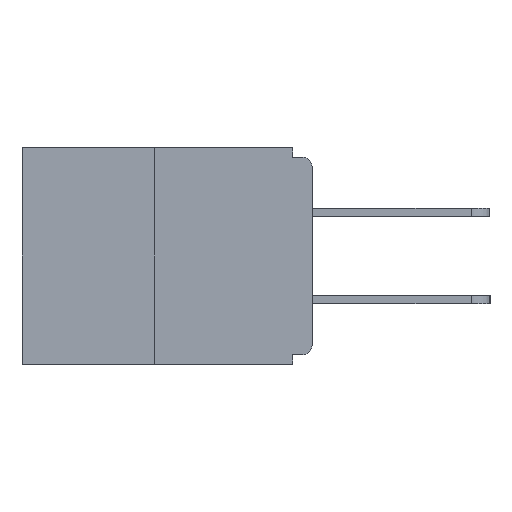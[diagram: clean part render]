
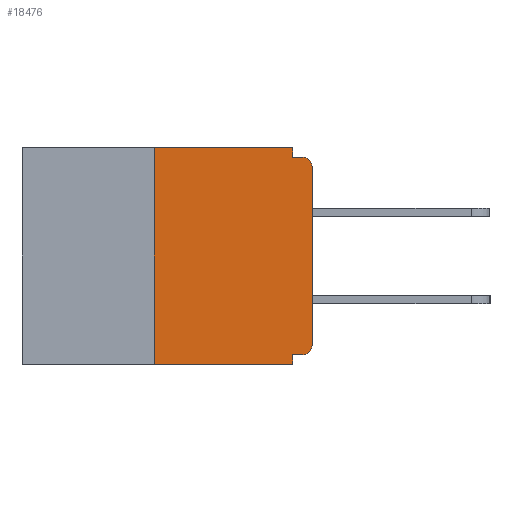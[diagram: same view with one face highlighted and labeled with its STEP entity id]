
A CAD part, left-side view. The second image highlights one B-rep face of the part: STEP entity #18476.
In plain terms, the highlighted planar face has unit normal (-1, 0, 0).
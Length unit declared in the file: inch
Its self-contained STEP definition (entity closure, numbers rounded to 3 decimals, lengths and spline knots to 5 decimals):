
#131 = EDGE_CURVE ( 'NONE', #29105, #17084, #5404, .T. ) ;
#136 = CARTESIAN_POINT ( 'NONE',  ( 0., 0.031, -0.343 ) ) ;
#494 = EDGE_CURVE ( 'NONE', #11780, #4640, #24787, .T. ) ;
#502 = VERTEX_POINT ( 'NONE', #136 ) ;
#1142 = CARTESIAN_POINT ( 'NONE',  ( 0., 0.25, -0.343 ) ) ;
#2443 = VECTOR ( 'NONE', #16193, 39.37008 ) ;
#2711 = CIRCLE ( 'NONE', #31239, 0.015 ) ;
#2719 = AXIS2_PLACEMENT_3D ( 'NONE', #22281, #15550, #10317 ) ;
#2957 = CARTESIAN_POINT ( 'NONE',  ( 0., 0.015, -0.015 ) ) ;
#4151 = VERTEX_POINT ( 'NONE', #19527 ) ;
#4197 = DIRECTION ( 'NONE',  ( 0., 1., 0. ) ) ;
#4585 = LINE ( 'NONE', #31349, #31183 ) ;
#4640 = VERTEX_POINT ( 'NONE', #27849 ) ;
#5404 = LINE ( 'NONE', #24868, #15585 ) ;
#5743 = ORIENTED_EDGE ( 'NONE', *, *, #494, .T. ) ;
#6564 = EDGE_CURVE ( 'NONE', #17084, #4151, #4585, .T. ) ;
#6596 = EDGE_CURVE ( 'NONE', #4640, #14128, #23706, .T. ) ;
#6706 = VERTEX_POINT ( 'NONE', #2957 ) ;
#7987 = VECTOR ( 'NONE', #19180, 39.37008 ) ;
#8022 = ORIENTED_EDGE ( 'NONE', *, *, #24861, .F. ) ;
#8413 = CARTESIAN_POINT ( 'NONE',  ( 0., 0., -0.03 ) ) ;
#8784 = ORIENTED_EDGE ( 'NONE', *, *, #8794, .T. ) ;
#8794 = EDGE_CURVE ( 'NONE', #19046, #502, #14116, .T. ) ;
#9097 = ORIENTED_EDGE ( 'NONE', *, *, #11865, .T. ) ;
#9131 = CARTESIAN_POINT ( 'NONE',  ( 0., 0.031, -0.343 ) ) ;
#10240 = DIRECTION ( 'NONE',  ( 0., 0., -1. ) ) ;
#10317 = DIRECTION ( 'NONE',  ( 0., 0., -1. ) ) ;
#11246 = VERTEX_POINT ( 'NONE', #11275 ) ;
#11275 = CARTESIAN_POINT ( 'NONE',  ( 0., 0.031, -0.328 ) ) ;
#11780 = VERTEX_POINT ( 'NONE', #12622 ) ;
#11865 = EDGE_CURVE ( 'NONE', #14128, #6706, #2711, .T. ) ;
#12084 = DIRECTION ( 'NONE',  ( -1., 0., 0. ) ) ;
#12622 = CARTESIAN_POINT ( 'NONE',  ( 0., 0.015, -0.328 ) ) ;
#13083 = VECTOR ( 'NONE', #30305, 39.37008 ) ;
#13108 = LINE ( 'NONE', #20452, #13083 ) ;
#13366 = VECTOR ( 'NONE', #28977, 39.37008 ) ;
#14116 = LINE ( 'NONE', #28466, #2443 ) ;
#14128 = VERTEX_POINT ( 'NONE', #8413 ) ;
#14313 = DIRECTION ( 'NONE',  ( 0., 0., -1. ) ) ;
#14617 = ORIENTED_EDGE ( 'NONE', *, *, #15140, .F. ) ;
#15140 = EDGE_CURVE ( 'NONE', #11780, #11246, #16648, .T. ) ;
#15550 = DIRECTION ( 'NONE',  ( 1., 0., 0. ) ) ;
#15585 = VECTOR ( 'NONE', #17389, 39.37008 ) ;
#16193 = DIRECTION ( 'NONE',  ( 0., -1., 0. ) ) ;
#16470 = LINE ( 'NONE', #9131, #19820 ) ;
#16648 = LINE ( 'NONE', #26533, #16731 ) ;
#16703 = CARTESIAN_POINT ( 'NONE',  ( 0., 0.25, 0. ) ) ;
#16731 = VECTOR ( 'NONE', #4197, 39.37008 ) ;
#17084 = VERTEX_POINT ( 'NONE', #29223 ) ;
#17389 = DIRECTION ( 'NONE',  ( 0., -1., 0. ) ) ;
#18476 = ADVANCED_FACE ( 'NONE', ( #27677 ), #22730, .F. ) ;
#19046 = VERTEX_POINT ( 'NONE', #1142 ) ;
#19180 = DIRECTION ( 'NONE',  ( 0., 0., 1. ) ) ;
#19527 = CARTESIAN_POINT ( 'NONE',  ( 0., 0.031, -0.015 ) ) ;
#19820 = VECTOR ( 'NONE', #21086, 39.37008 ) ;
#20452 = CARTESIAN_POINT ( 'NONE',  ( 0., 0., -0.015 ) ) ;
#21086 = DIRECTION ( 'NONE',  ( 0., 0., -1. ) ) ;
#21626 = EDGE_LOOP ( 'NONE', ( #28104, #25521, #8784, #8022, #14617, #5743, #24420, #9097, #30937, #31220 ) ) ;
#22281 = CARTESIAN_POINT ( 'NONE',  ( 0., 0.46, 0. ) ) ;
#22730 = PLANE ( 'NONE',  #2719 ) ;
#23474 = LINE ( 'NONE', #31281, #7987 ) ;
#23706 = LINE ( 'NONE', #31196, #13366 ) ;
#23731 = EDGE_CURVE ( 'NONE', #19046, #29105, #23474, .T. ) ;
#24420 = ORIENTED_EDGE ( 'NONE', *, *, #6596, .T. ) ;
#24722 = CARTESIAN_POINT ( 'NONE',  ( 0., 0.015, -0.03 ) ) ;
#24787 = CIRCLE ( 'NONE', #28866, 0.015 ) ;
#24861 = EDGE_CURVE ( 'NONE', #11246, #502, #16470, .T. ) ;
#24868 = CARTESIAN_POINT ( 'NONE',  ( 0., 0.46, 0. ) ) ;
#24893 = DIRECTION ( 'NONE',  ( -1., 0., 0. ) ) ;
#25521 = ORIENTED_EDGE ( 'NONE', *, *, #23731, .F. ) ;
#26264 = CARTESIAN_POINT ( 'NONE',  ( 0., 0.015, -0.313 ) ) ;
#26533 = CARTESIAN_POINT ( 'NONE',  ( 0., 0., -0.328 ) ) ;
#27677 = FACE_OUTER_BOUND ( 'NONE', #21626, .T. ) ;
#27849 = CARTESIAN_POINT ( 'NONE',  ( 0., 0., -0.313 ) ) ;
#28104 = ORIENTED_EDGE ( 'NONE', *, *, #131, .F. ) ;
#28466 = CARTESIAN_POINT ( 'NONE',  ( 0., 0.46, -0.343 ) ) ;
#28496 = EDGE_CURVE ( 'NONE', #4151, #6706, #13108, .T. ) ;
#28866 = AXIS2_PLACEMENT_3D ( 'NONE', #26264, #12084, #28997 ) ;
#28977 = DIRECTION ( 'NONE',  ( 0., 0., 1. ) ) ;
#28997 = DIRECTION ( 'NONE',  ( 0., 0., -1. ) ) ;
#29105 = VERTEX_POINT ( 'NONE', #16703 ) ;
#29223 = CARTESIAN_POINT ( 'NONE',  ( 0., 0.031, 0. ) ) ;
#30305 = DIRECTION ( 'NONE',  ( 0., -1., 0. ) ) ;
#30937 = ORIENTED_EDGE ( 'NONE', *, *, #28496, .F. ) ;
#31183 = VECTOR ( 'NONE', #14313, 39.37008 ) ;
#31196 = CARTESIAN_POINT ( 'NONE',  ( 0., 0., 0. ) ) ;
#31220 = ORIENTED_EDGE ( 'NONE', *, *, #6564, .F. ) ;
#31239 = AXIS2_PLACEMENT_3D ( 'NONE', #24722, #24893, #10240 ) ;
#31281 = CARTESIAN_POINT ( 'NONE',  ( 0., 0.25, 0. ) ) ;
#31349 = CARTESIAN_POINT ( 'NONE',  ( 0., 0.031, 0. ) ) ;
